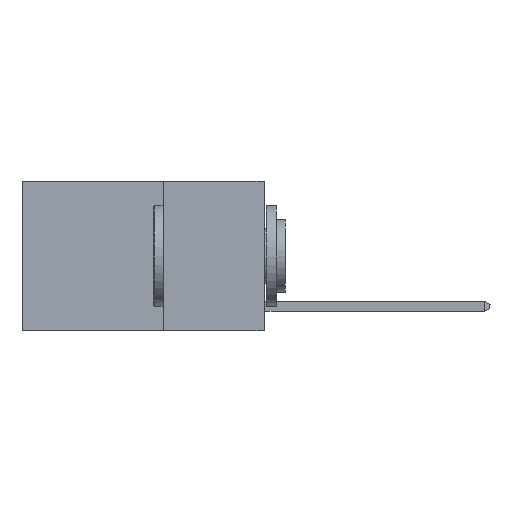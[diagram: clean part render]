
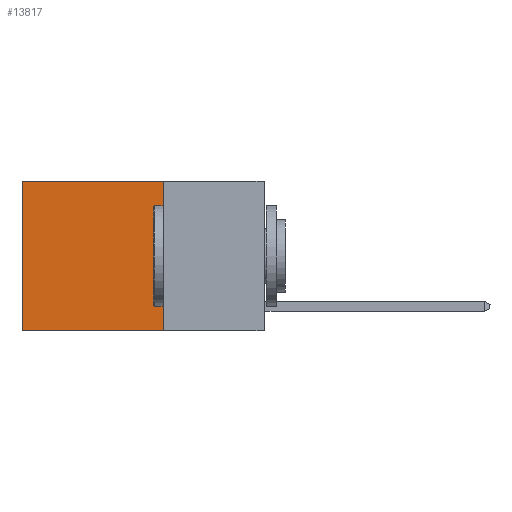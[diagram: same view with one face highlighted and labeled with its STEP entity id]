
A CAD part, left-side view. The second image highlights one B-rep face of the part: STEP entity #13817.
In plain terms, the highlighted planar face has unit normal (-1, 0, 0).
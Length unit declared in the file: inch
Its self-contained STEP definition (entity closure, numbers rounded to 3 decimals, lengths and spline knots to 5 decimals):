
#1016 = LINE ( 'NONE', #16672, #15736 ) ;
#1073 = ORIENTED_EDGE ( 'NONE', *, *, #9702, .F. ) ;
#1471 = CARTESIAN_POINT ( 'NONE',  ( 0.2625, 0.25, 0. ) ) ;
#2346 = PLANE ( 'NONE',  #19237 ) ;
#3960 = LINE ( 'NONE', #1471, #23666 ) ;
#4229 = CARTESIAN_POINT ( 'NONE',  ( 0.2625, 0.25, -0.37 ) ) ;
#4305 = DIRECTION ( 'NONE',  ( 0., 0., -1. ) ) ;
#4558 = ORIENTED_EDGE ( 'NONE', *, *, #21424, .T. ) ;
#4909 = EDGE_LOOP ( 'NONE', ( #4558, #19372, #1073, #15863 ) ) ;
#8970 = LINE ( 'NONE', #23753, #23022 ) ;
#9452 = VERTEX_POINT ( 'NONE', #21897 ) ;
#9702 = EDGE_CURVE ( 'NONE', #9452, #20899, #3960, .T. ) ;
#10411 = DIRECTION ( 'NONE',  ( 0., 1., 0. ) ) ;
#10890 = CARTESIAN_POINT ( 'NONE',  ( 0.2625, 0.6, -0.37 ) ) ;
#13612 = CARTESIAN_POINT ( 'NONE',  ( 0.2625, 0.6, 0. ) ) ;
#13765 = DIRECTION ( 'NONE',  ( 0., 1., 0. ) ) ;
#13817 = ADVANCED_FACE ( 'NONE', ( #23505 ), #2346, .F. ) ;
#14667 = VECTOR ( 'NONE', #13765, 39.37008 ) ;
#14837 = DIRECTION ( 'NONE',  ( 0., 0., -1. ) ) ;
#15736 = VECTOR ( 'NONE', #14837, 39.37008 ) ;
#15763 = DIRECTION ( 'NONE',  ( 1., 0., 0. ) ) ;
#15863 = ORIENTED_EDGE ( 'NONE', *, *, #18448, .T. ) ;
#16672 = CARTESIAN_POINT ( 'NONE',  ( 0.2625, 0.6, 0. ) ) ;
#16810 = DIRECTION ( 'NONE',  ( 0., 0., -1. ) ) ;
#16911 = VERTEX_POINT ( 'NONE', #10890 ) ;
#18285 = VERTEX_POINT ( 'NONE', #13612 ) ;
#18448 = EDGE_CURVE ( 'NONE', #9452, #18285, #8970, .T. ) ;
#18854 = EDGE_CURVE ( 'NONE', #20899, #16911, #24800, .T. ) ;
#19042 = CARTESIAN_POINT ( 'NONE',  ( 0.2625, 0.25, -0.37 ) ) ;
#19237 = AXIS2_PLACEMENT_3D ( 'NONE', #21419, #15763, #4305 ) ;
#19372 = ORIENTED_EDGE ( 'NONE', *, *, #18854, .F. ) ;
#20899 = VERTEX_POINT ( 'NONE', #19042 ) ;
#21419 = CARTESIAN_POINT ( 'NONE',  ( 0.2625, 0.25, 0. ) ) ;
#21424 = EDGE_CURVE ( 'NONE', #18285, #16911, #1016, .T. ) ;
#21897 = CARTESIAN_POINT ( 'NONE',  ( 0.2625, 0.25, 0. ) ) ;
#23022 = VECTOR ( 'NONE', #10411, 39.37008 ) ;
#23505 = FACE_OUTER_BOUND ( 'NONE', #4909, .T. ) ;
#23666 = VECTOR ( 'NONE', #16810, 39.37008 ) ;
#23753 = CARTESIAN_POINT ( 'NONE',  ( 0.2625, 0.25, 0. ) ) ;
#24800 = LINE ( 'NONE', #4229, #14667 ) ;
